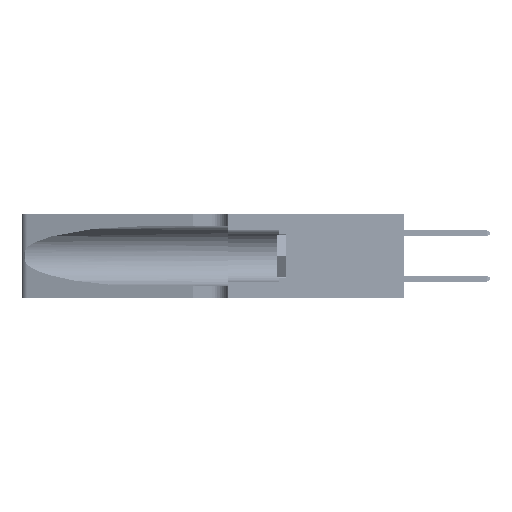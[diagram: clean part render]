
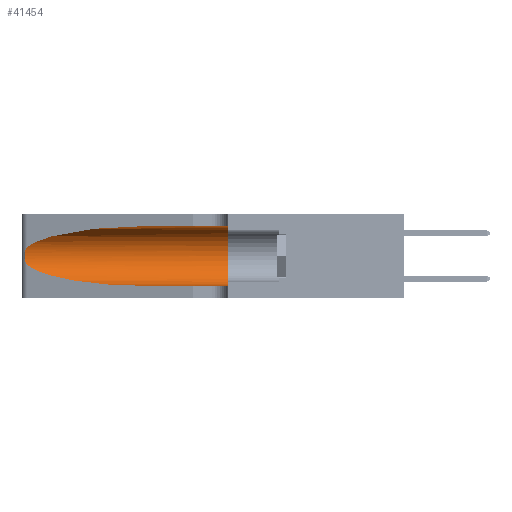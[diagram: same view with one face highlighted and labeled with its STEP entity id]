
A CAD part, left-side view. The second image highlights one B-rep face of the part: STEP entity #41454.
In plain terms, the highlighted cylindrical face has radius 3.308 mm (diameter 6.617 mm), a partial arc.
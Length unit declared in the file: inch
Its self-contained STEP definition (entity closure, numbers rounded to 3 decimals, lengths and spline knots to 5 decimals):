
#1468 = VERTEX_POINT ( 'NONE', #14252 ) ;
#3057 = EDGE_CURVE ( 'NONE', #39308, #32618, #13715, .T. ) ;
#3154 = CARTESIAN_POINT ( 'NONE',  ( 0.1305, 0.72297, 0.31525 ) ) ;
#3233 = CARTESIAN_POINT ( 'NONE',  ( 0.25787, 1.23484, 0.2124 ) ) ;
#3314 = CARTESIAN_POINT ( 'NONE',  ( 0.2373, 1.15595, 0.28018 ) ) ;
#3571 = B_SPLINE_CURVE_WITH_KNOTS ( 'NONE', 3,
 ( #49085, #37649, #26116, #3233, #30110, #7116, #33981, #10973, #37818, #14873, #41623, #18756, #45425, #22611 ),
 .UNSPECIFIED., .F., .F.,
 ( 4, 2, 2, 2, 2, 2, 4 ),
 ( 0., 0.00027, 0.00053, 0.00107, 0.0016, 0.00187, 0.00214 ),
 .UNSPECIFIED. ) ;
#4207 = DIRECTION ( 'NONE',  ( 0., 1., 0. ) ) ;
#6230 = CARTESIAN_POINT ( 'NONE',  ( 0.1305, 1.61858, 0.05475 ) ) ;
#7116 = CARTESIAN_POINT ( 'NONE',  ( 0.26018, 1.23835, 0.19895 ) ) ;
#7181 = ORIENTED_EDGE ( 'NONE', *, *, #37015, .T. ) ;
#7944 = VECTOR ( 'NONE', #10102, 39.37008 ) ;
#8655 = DIRECTION ( 'NONE',  ( 0., -1., 0. ) ) ;
#10058 = ORIENTED_EDGE ( 'NONE', *, *, #3057, .F. ) ;
#10102 = DIRECTION ( 'NONE',  ( 0., -1., 0. ) ) ;
#10889 = CARTESIAN_POINT ( 'NONE',  ( 0.18966, 0.96281, 0.31525 ) ) ;
#10973 = CARTESIAN_POINT ( 'NONE',  ( 0.26075, 1.23896, 0.178 ) ) ;
#13715 = CIRCLE ( 'NONE', #44576, 0.13025 ) ;
#14252 = CARTESIAN_POINT ( 'NONE',  ( 0.1305, 0.72297, 0.05475 ) ) ;
#14873 = CARTESIAN_POINT ( 'NONE',  ( 0.25856, 1.23593, 0.16098 ) ) ;
#15641 = ORIENTED_EDGE ( 'NONE', *, *, #18341, .T. ) ;
#15657 = CARTESIAN_POINT ( 'NONE',  ( 0.25487, 1.22718, 0.14631 ) ) ;
#16407 = CARTESIAN_POINT ( 'NONE',  ( 0.1305, 1.61858, 0.185 ) ) ;
#17493 = ORIENTED_EDGE ( 'NONE', *, *, #47912, .T. ) ;
#17794 =( BOUNDED_CURVE ( )  B_SPLINE_CURVE ( 3, ( #48733, #22092, #41283, #18396 ),
 .UNSPECIFIED., .F., .F. ) 
 B_SPLINE_CURVE_WITH_KNOTS ( ( 4, 4 ),
 ( 3.44316, 4.71239 ),
 .UNSPECIFIED. ) 
 CURVE ( )  GEOMETRIC_REPRESENTATION_ITEM ( )  RATIONAL_B_SPLINE_CURVE ( ( 1., 0.87, 0.87, 1. ) ) 
 REPRESENTATION_ITEM ( '' )  );
#18201 = LINE ( 'NONE', #6230, #7944 ) ;
#18341 = EDGE_CURVE ( 'NONE', #36739, #40628, #3571, .T. ) ;
#18396 = CARTESIAN_POINT ( 'NONE',  ( 0.1305, 0.72297, 0.05475 ) ) ;
#18756 = CARTESIAN_POINT ( 'NONE',  ( 0.25639, 1.23186, 0.15144 ) ) ;
#18888 = DIRECTION ( 'NONE',  ( 0., -1., 0. ) ) ;
#21461 = ORIENTED_EDGE ( 'NONE', *, *, #45363, .F. ) ;
#22092 = CARTESIAN_POINT ( 'NONE',  ( 0.2373, 1.15595, 0.08982 ) ) ;
#22611 = CARTESIAN_POINT ( 'NONE',  ( 0.25487, 1.22718, 0.14631 ) ) ;
#24131 = CYLINDRICAL_SURFACE ( 'NONE', #26645, 0.13025 ) ;
#26116 = CARTESIAN_POINT ( 'NONE',  ( 0.25639, 1.23184, 0.21858 ) ) ;
#26645 = AXIS2_PLACEMENT_3D ( 'NONE', #16407, #8655, #43145 ) ;
#27239 = CARTESIAN_POINT ( 'NONE',  ( 0.1305, 0.35, 0.185 ) ) ;
#29082 = CARTESIAN_POINT ( 'NONE',  ( 0.1305, 0.72297, 0.31525 ) ) ;
#30110 = CARTESIAN_POINT ( 'NONE',  ( 0.25854, 1.2359, 0.20912 ) ) ;
#30197 = CARTESIAN_POINT ( 'NONE',  ( 0.25487, 1.22718, 0.22369 ) ) ;
#30411 = CARTESIAN_POINT ( 'NONE',  ( 0.1305, 1.61858, 0.31525 ) ) ;
#30502 = VERTEX_POINT ( 'NONE', #29082 ) ;
#31098 = DIRECTION ( 'NONE',  ( 0., 0., 1. ) ) ;
#32618 = VERTEX_POINT ( 'NONE', #41445 ) ;
#33981 = CARTESIAN_POINT ( 'NONE',  ( 0.26075, 1.23896, 0.19203 ) ) ;
#36739 = VERTEX_POINT ( 'NONE', #39125 ) ;
#37015 = EDGE_CURVE ( 'NONE', #1468, #32618, #18201, .T. ) ;
#37649 = CARTESIAN_POINT ( 'NONE',  ( 0.25555, 1.22994, 0.2215 ) ) ;
#37818 = CARTESIAN_POINT ( 'NONE',  ( 0.26017, 1.23833, 0.17102 ) ) ;
#38522 = ORIENTED_EDGE ( 'NONE', *, *, #39838, .T. ) ;
#39125 = CARTESIAN_POINT ( 'NONE',  ( 0.25487, 1.22718, 0.22369 ) ) ;
#39308 = VERTEX_POINT ( 'NONE', #45793 ) ;
#39838 = EDGE_CURVE ( 'NONE', #40628, #1468, #17794, .T. ) ;
#40628 = VERTEX_POINT ( 'NONE', #15657 ) ;
#40755 =( BOUNDED_CURVE ( )  B_SPLINE_CURVE ( 3, ( #3154, #10889, #3314, #30197 ),
 .UNSPECIFIED., .F., .F. ) 
 B_SPLINE_CURVE_WITH_KNOTS ( ( 4, 4 ),
 ( 1.5708, 2.84003 ),
 .UNSPECIFIED. ) 
 CURVE ( )  GEOMETRIC_REPRESENTATION_ITEM ( )  RATIONAL_B_SPLINE_CURVE ( ( 1., 0.87, 0.87, 1. ) ) 
 REPRESENTATION_ITEM ( '' )  );
#41283 = CARTESIAN_POINT ( 'NONE',  ( 0.18966, 0.96281, 0.05475 ) ) ;
#41445 = CARTESIAN_POINT ( 'NONE',  ( 0.1305, 0.35, 0.05475 ) ) ;
#41454 = ADVANCED_FACE ( 'NONE', ( #44388 ), #24131, .F. ) ;
#41623 = CARTESIAN_POINT ( 'NONE',  ( 0.25789, 1.23486, 0.15765 ) ) ;
#43145 = DIRECTION ( 'NONE',  ( 0., 0., -1. ) ) ;
#44388 = FACE_OUTER_BOUND ( 'NONE', #45385, .T. ) ;
#44576 = AXIS2_PLACEMENT_3D ( 'NONE', #27239, #4207, #31098 ) ;
#45363 = EDGE_CURVE ( 'NONE', #30502, #39308, #47010, .T. ) ;
#45385 = EDGE_LOOP ( 'NONE', ( #17493, #15641, #38522, #7181, #10058, #21461 ) ) ;
#45425 = CARTESIAN_POINT ( 'NONE',  ( 0.25555, 1.22993, 0.14849 ) ) ;
#45793 = CARTESIAN_POINT ( 'NONE',  ( 0.1305, 0.35, 0.31525 ) ) ;
#45836 = VECTOR ( 'NONE', #18888, 39.37008 ) ;
#47010 = LINE ( 'NONE', #30411, #45836 ) ;
#47912 = EDGE_CURVE ( 'NONE', #30502, #36739, #40755, .T. ) ;
#48733 = CARTESIAN_POINT ( 'NONE',  ( 0.25487, 1.22718, 0.14631 ) ) ;
#49085 = CARTESIAN_POINT ( 'NONE',  ( 0.25487, 1.22718, 0.22369 ) ) ;
